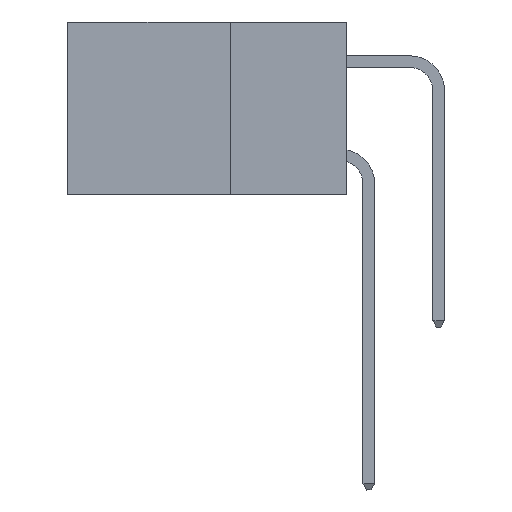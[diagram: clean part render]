
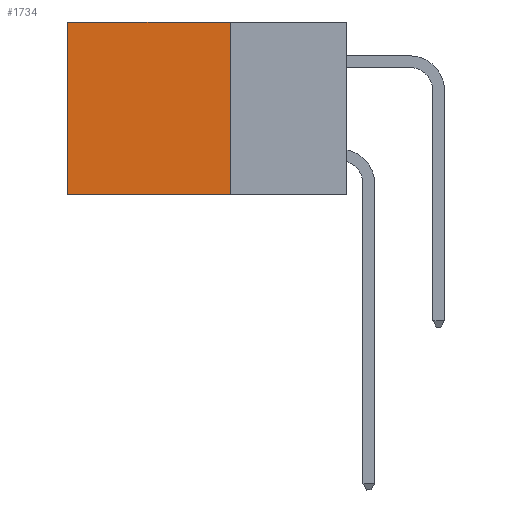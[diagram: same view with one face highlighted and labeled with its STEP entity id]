
A CAD part, left-side view. The second image highlights one B-rep face of the part: STEP entity #1734.
In plain terms, the highlighted planar face has unit normal (-1, 0, 0).
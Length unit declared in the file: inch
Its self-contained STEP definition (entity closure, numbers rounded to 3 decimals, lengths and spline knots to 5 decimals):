
#1485 = EDGE_CURVE ( 'NONE', #25193, #9095, #10753, .T. ) ;
#1734 = ADVANCED_FACE ( 'NONE', ( #22877 ), #17550, .F. ) ;
#4742 = VECTOR ( 'NONE', #25784, 39.37008 ) ;
#7048 = EDGE_CURVE ( 'NONE', #19355, #9095, #20547, .T. ) ;
#7462 = ORIENTED_EDGE ( 'NONE', *, *, #7048, .T. ) ;
#8506 = CARTESIAN_POINT ( 'NONE',  ( 0.2875, 0.25, -0.37 ) ) ;
#8685 = CARTESIAN_POINT ( 'NONE',  ( 0.2875, 0.25, 0. ) ) ;
#9020 = ORIENTED_EDGE ( 'NONE', *, *, #15862, .F. ) ;
#9095 = VERTEX_POINT ( 'NONE', #20702 ) ;
#10753 = LINE ( 'NONE', #8506, #21446 ) ;
#11271 = DIRECTION ( 'NONE',  ( 1., 0., 0. ) ) ;
#11664 = AXIS2_PLACEMENT_3D ( 'NONE', #8685, #11271, #38114 ) ;
#15862 = EDGE_CURVE ( 'NONE', #19970, #25193, #29918, .T. ) ;
#17338 = CARTESIAN_POINT ( 'NONE',  ( 0.2875, 0.6, 0. ) ) ;
#17550 = PLANE ( 'NONE',  #11664 ) ;
#18277 = VECTOR ( 'NONE', #22825, 39.37008 ) ;
#18999 = CARTESIAN_POINT ( 'NONE',  ( 0.2875, 0.25, 0. ) ) ;
#19355 = VERTEX_POINT ( 'NONE', #30662 ) ;
#19970 = VERTEX_POINT ( 'NONE', #18999 ) ;
#20547 = LINE ( 'NONE', #17338, #4742 ) ;
#20702 = CARTESIAN_POINT ( 'NONE',  ( 0.2875, 0.6, -0.37 ) ) ;
#21243 = CARTESIAN_POINT ( 'NONE',  ( 0.2875, 0.25, 0. ) ) ;
#21446 = VECTOR ( 'NONE', #31659, 39.37008 ) ;
#22825 = DIRECTION ( 'NONE',  ( 0., 0., -1. ) ) ;
#22877 = FACE_OUTER_BOUND ( 'NONE', #32203, .T. ) ;
#25193 = VERTEX_POINT ( 'NONE', #29011 ) ;
#25784 = DIRECTION ( 'NONE',  ( 0., 0., -1. ) ) ;
#27209 = DIRECTION ( 'NONE',  ( 0., 1., 0. ) ) ;
#27624 = LINE ( 'NONE', #21243, #31373 ) ;
#28924 = CARTESIAN_POINT ( 'NONE',  ( 0.2875, 0.25, 0. ) ) ;
#29011 = CARTESIAN_POINT ( 'NONE',  ( 0.2875, 0.25, -0.37 ) ) ;
#29918 = LINE ( 'NONE', #28924, #18277 ) ;
#30045 = ORIENTED_EDGE ( 'NONE', *, *, #37588, .T. ) ;
#30662 = CARTESIAN_POINT ( 'NONE',  ( 0.2875, 0.6, 0. ) ) ;
#31373 = VECTOR ( 'NONE', #27209, 39.37008 ) ;
#31659 = DIRECTION ( 'NONE',  ( 0., 1., 0. ) ) ;
#32203 = EDGE_LOOP ( 'NONE', ( #7462, #38364, #9020, #30045 ) ) ;
#37588 = EDGE_CURVE ( 'NONE', #19970, #19355, #27624, .T. ) ;
#38114 = DIRECTION ( 'NONE',  ( 0., 0., -1. ) ) ;
#38364 = ORIENTED_EDGE ( 'NONE', *, *, #1485, .F. ) ;
